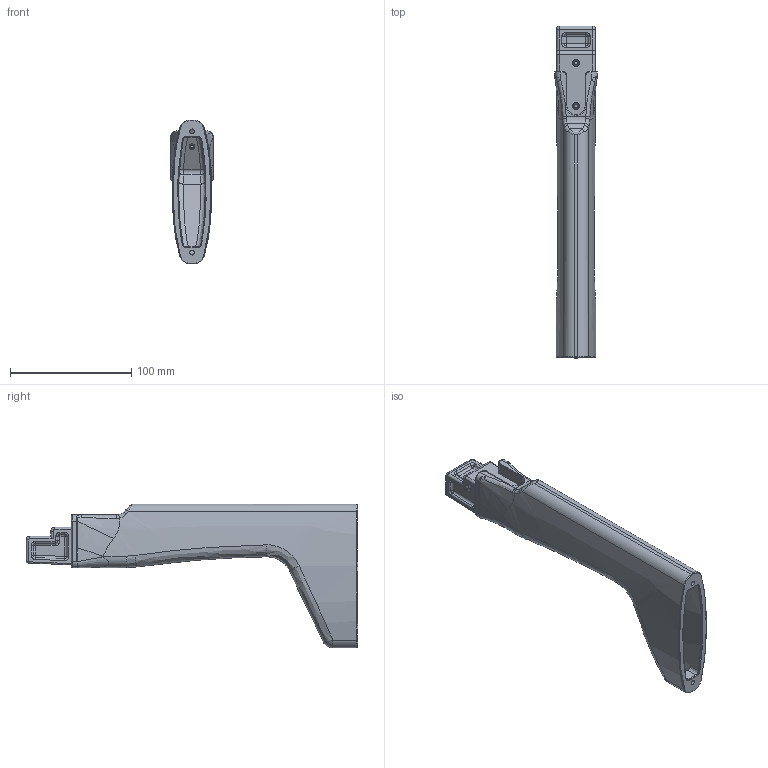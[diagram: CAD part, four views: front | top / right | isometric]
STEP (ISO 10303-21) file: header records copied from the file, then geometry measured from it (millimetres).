
FILE_DESCRIPTION(/* description */ (''),/* implementation_level */ '2;1');
FILE_NAME(/* name */ 'Full Stock Body.step',/* time_stamp */ '2021-10-03T07:01:06-04:00',/* author */ (''),/* organization */ (''),/* preprocessor_version */ 'ST-DEVELOPER v18.1',/* originating_system */ 'Autodesk Translation Framework v10.10.0.1391',/* authorisation */ '');
FILE_SCHEMA (('AUTOMOTIVE_DESIGN { 1 0 10303 214 3 1 1 }'));
Length unit declared in the file: millimetre
Products named in the file (1): 1 Piece Stock
Bounding box: 35 x 273.35 x 118.61 mm (x, y, z)
Volume: 230247.4 mm3; surface area: 73688.9 mm2
Topology: 1 solids, 1 shells, 413 faces, 931 edges, 529 vertices
Faces by surface type: bspline 171, cylinder 122, plane 45, torus 39, sphere 30, cone 6
Full cylindrical faces by diameter (mm): 2.636 x2, 3.8 x2, 4.6 x2
Entity records: 16601 total; most frequent: CARTESIAN_POINT 8205, ORIENTED_EDGE 1846, DIRECTION 1545, EDGE_CURVE 923, AXIS2_PLACEMENT_3D 645, VERTEX_POINT 529, EDGE_LOOP 434, FACE_OUTER_BOUND 413
